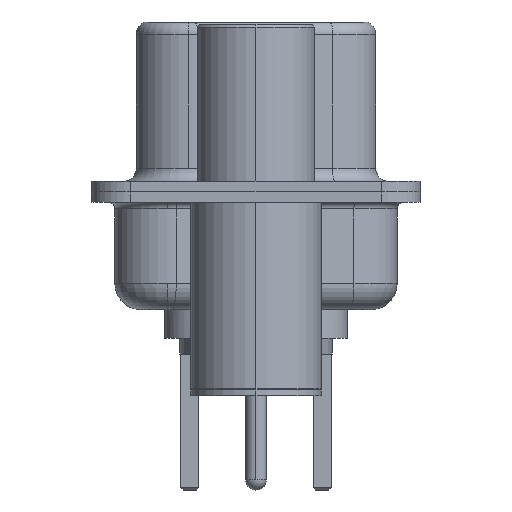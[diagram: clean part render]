
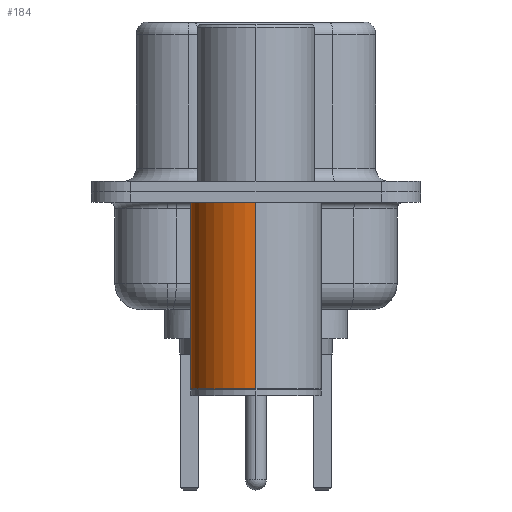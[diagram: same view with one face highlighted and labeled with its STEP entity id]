
A CAD part, left-side view. The second image highlights one B-rep face of the part: STEP entity #184.
In plain terms, the highlighted cylindrical face has radius 2.5 mm (diameter 5 mm), a partial arc.
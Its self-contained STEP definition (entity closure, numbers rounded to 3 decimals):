
#184 = ADVANCED_FACE ( 'NONE', ( #4960 ), #12160, .T. ) ;
#1180 = VERTEX_POINT ( 'NONE', #17936 ) ;
#1699 = CARTESIAN_POINT ( 'NONE',  ( 2.5, 0., -0.4 ) ) ;
#2721 = CARTESIAN_POINT ( 'NONE',  ( 0., 0., -0.4 ) ) ;
#3904 = EDGE_CURVE ( 'NONE', #18263, #7095, #16038, .T. ) ;
#4138 = DIRECTION ( 'NONE',  ( 1., 0., 0. ) ) ;
#4567 = ORIENTED_EDGE ( 'NONE', *, *, #18679, .T. ) ;
#4721 = LINE ( 'NONE', #11942, #12357 ) ;
#4960 = FACE_OUTER_BOUND ( 'NONE', #13929, .T. ) ;
#5831 = CARTESIAN_POINT ( 'NONE',  ( 0., 0., -7.525 ) ) ;
#5855 = DIRECTION ( 'NONE',  ( 0., 0., 1. ) ) ;
#6948 = DIRECTION ( 'NONE',  ( 1., 0., 0. ) ) ;
#7005 = EDGE_CURVE ( 'NONE', #18358, #1180, #12308, .T. ) ;
#7095 = VERTEX_POINT ( 'NONE', #16662 ) ;
#7207 = CARTESIAN_POINT ( 'NONE',  ( 2.5, 0., -7.525 ) ) ;
#7783 = CARTESIAN_POINT ( 'NONE',  ( -2.5, 0., 0.581 ) ) ;
#8975 = DIRECTION ( 'NONE',  ( 0., 0., 1. ) ) ;
#9101 = CARTESIAN_POINT ( 'NONE',  ( 0., 0., 0.581 ) ) ;
#9205 = DIRECTION ( 'NONE',  ( 0., 0., 1. ) ) ;
#11497 = AXIS2_PLACEMENT_3D ( 'NONE', #2721, #12762, #4138 ) ;
#11850 = ORIENTED_EDGE ( 'NONE', *, *, #3904, .T. ) ;
#11942 = CARTESIAN_POINT ( 'NONE',  ( 2.5, 0., 0.581 ) ) ;
#12044 = LINE ( 'NONE', #7783, #15451 ) ;
#12160 = CYLINDRICAL_SURFACE ( 'NONE', #17756, 2.5 ) ;
#12308 = CIRCLE ( 'NONE', #11497, 2.5 ) ;
#12357 = VECTOR ( 'NONE', #16250, 1000. ) ;
#12762 = DIRECTION ( 'NONE',  ( 0., 0., 1. ) ) ;
#13929 = EDGE_LOOP ( 'NONE', ( #11850, #4567, #16825, #18802 ) ) ;
#14651 = DIRECTION ( 'NONE',  ( 1., 0., 0. ) ) ;
#15451 = VECTOR ( 'NONE', #9205, 1000. ) ;
#16038 = CIRCLE ( 'NONE', #17443, 2.5 ) ;
#16250 = DIRECTION ( 'NONE',  ( 0., 0., 1. ) ) ;
#16662 = CARTESIAN_POINT ( 'NONE',  ( -2.5, 0., -7.525 ) ) ;
#16825 = ORIENTED_EDGE ( 'NONE', *, *, #7005, .F. ) ;
#17174 = EDGE_CURVE ( 'NONE', #18263, #18358, #4721, .T. ) ;
#17443 = AXIS2_PLACEMENT_3D ( 'NONE', #5831, #5855, #6948 ) ;
#17756 = AXIS2_PLACEMENT_3D ( 'NONE', #9101, #8975, #14651 ) ;
#17936 = CARTESIAN_POINT ( 'NONE',  ( -2.5, 0., -0.4 ) ) ;
#18263 = VERTEX_POINT ( 'NONE', #7207 ) ;
#18358 = VERTEX_POINT ( 'NONE', #1699 ) ;
#18679 = EDGE_CURVE ( 'NONE', #7095, #1180, #12044, .T. ) ;
#18802 = ORIENTED_EDGE ( 'NONE', *, *, #17174, .F. ) ;
